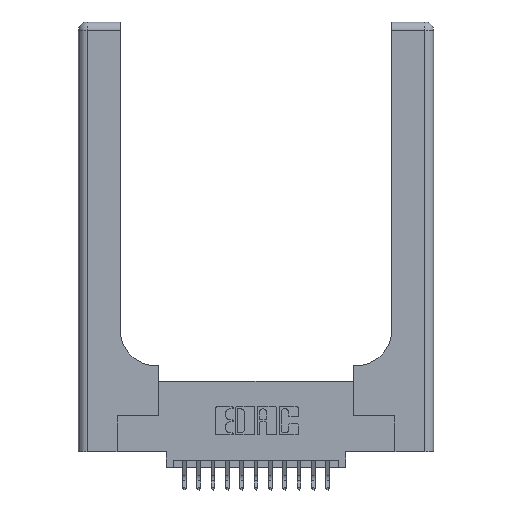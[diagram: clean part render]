
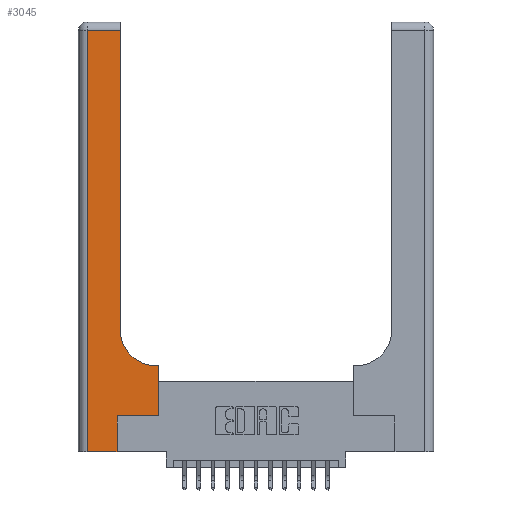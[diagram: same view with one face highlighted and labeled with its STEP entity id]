
A CAD part, top view. The second image highlights one B-rep face of the part: STEP entity #3045.
In plain terms, the highlighted planar face has unit normal (0, 0, 1).
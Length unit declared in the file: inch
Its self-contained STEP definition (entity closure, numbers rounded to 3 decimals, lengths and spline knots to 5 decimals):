
#62 = EDGE_CURVE ( 'NONE', #556, #14272, #10894, .T. ) ;
#209 = ORIENTED_EDGE ( 'NONE', *, *, #3228, .T. ) ;
#393 = ORIENTED_EDGE ( 'NONE', *, *, #5946, .T. ) ;
#556 = VERTEX_POINT ( 'NONE', #5649 ) ;
#720 = VERTEX_POINT ( 'NONE', #1015 ) ;
#737 = CARTESIAN_POINT ( 'NONE',  ( 0.269, 0.25, 0.37 ) ) ;
#1014 = LINE ( 'NONE', #6692, #4306 ) ;
#1015 = CARTESIAN_POINT ( 'NONE',  ( 0.5415, 0.6, 0.37 ) ) ;
#1060 = CARTESIAN_POINT ( 'NONE',  ( 0.06, 0., 0.37 ) ) ;
#1127 = CARTESIAN_POINT ( 'NONE',  ( 0., 3., 0.37 ) ) ;
#1320 = DIRECTION ( 'NONE',  ( -1., 0., 0. ) ) ;
#1428 = ORIENTED_EDGE ( 'NONE', *, *, #4785, .T. ) ;
#1470 = CARTESIAN_POINT ( 'NONE',  ( 0., 2.94, 0.37 ) ) ;
#2487 = LINE ( 'NONE', #14448, #9619 ) ;
#2597 = VECTOR ( 'NONE', #16921, 39.37008 ) ;
#3045 = ADVANCED_FACE ( 'NONE', ( #12782 ), #7620, .F. ) ;
#3191 = DIRECTION ( 'NONE',  ( 0., 1., 0. ) ) ;
#3228 = EDGE_CURVE ( 'NONE', #4507, #6204, #1014, .T. ) ;
#3285 = DIRECTION ( 'NONE',  ( 1., 0., 0. ) ) ;
#3406 = VECTOR ( 'NONE', #9528, 39.37008 ) ;
#3554 = ORIENTED_EDGE ( 'NONE', *, *, #9124, .T. ) ;
#3747 = LINE ( 'NONE', #6842, #15785 ) ;
#3970 = CARTESIAN_POINT ( 'NONE',  ( 0.2915, 0.85, 0.37 ) ) ;
#4130 = CARTESIAN_POINT ( 'NONE',  ( 0.269, 0., 0.37 ) ) ;
#4306 = VECTOR ( 'NONE', #12244, 39.37008 ) ;
#4507 = VERTEX_POINT ( 'NONE', #10800 ) ;
#4729 = LINE ( 'NONE', #10486, #10089 ) ;
#4785 = EDGE_CURVE ( 'NONE', #6204, #15119, #2487, .T. ) ;
#4969 = ORIENTED_EDGE ( 'NONE', *, *, #13671, .T. ) ;
#5626 = DIRECTION ( 'NONE',  ( 0., 0., -1. ) ) ;
#5649 = CARTESIAN_POINT ( 'NONE',  ( 0.269, 0.25, 0.37 ) ) ;
#5757 = CIRCLE ( 'NONE', #16967, 0.25 ) ;
#5946 = EDGE_CURVE ( 'NONE', #11064, #14195, #4729, .T. ) ;
#6022 = EDGE_LOOP ( 'NONE', ( #393, #6924, #209, #1428, #7996, #14332, #7759, #4969, #3554 ) ) ;
#6204 = VERTEX_POINT ( 'NONE', #1060 ) ;
#6692 = CARTESIAN_POINT ( 'NONE',  ( 0.06, 3., 0.37 ) ) ;
#6842 = CARTESIAN_POINT ( 'NONE',  ( 0.2915, 0.6, 0.37 ) ) ;
#6924 = ORIENTED_EDGE ( 'NONE', *, *, #10395, .T. ) ;
#7087 = VECTOR ( 'NONE', #14965, 39.37008 ) ;
#7620 = PLANE ( 'NONE',  #17017 ) ;
#7759 = ORIENTED_EDGE ( 'NONE', *, *, #17238, .T. ) ;
#7996 = ORIENTED_EDGE ( 'NONE', *, *, #16711, .T. ) ;
#9124 = EDGE_CURVE ( 'NONE', #720, #11064, #5757, .T. ) ;
#9528 = DIRECTION ( 'NONE',  ( 0., 1., 0. ) ) ;
#9619 = VECTOR ( 'NONE', #3285, 39.37008 ) ;
#10089 = VECTOR ( 'NONE', #11914, 39.37008 ) ;
#10395 = EDGE_CURVE ( 'NONE', #14195, #4507, #17939, .T. ) ;
#10486 = CARTESIAN_POINT ( 'NONE',  ( 0.2915, 3., 0.37 ) ) ;
#10800 = CARTESIAN_POINT ( 'NONE',  ( 0.06, 2.94, 0.37 ) ) ;
#10894 = LINE ( 'NONE', #737, #7087 ) ;
#11064 = VERTEX_POINT ( 'NONE', #3970 ) ;
#11742 = CARTESIAN_POINT ( 'NONE',  ( 0.5585, 0.25, 0.37 ) ) ;
#11914 = DIRECTION ( 'NONE',  ( 0., 1., 0. ) ) ;
#12244 = DIRECTION ( 'NONE',  ( 0., -1., 0. ) ) ;
#12433 = DIRECTION ( 'NONE',  ( 0., 0., -1. ) ) ;
#12497 = DIRECTION ( 'NONE',  ( 1., 0., 0. ) ) ;
#12782 = FACE_OUTER_BOUND ( 'NONE', #6022, .T. ) ;
#12825 = VERTEX_POINT ( 'NONE', #13288 ) ;
#13288 = CARTESIAN_POINT ( 'NONE',  ( 0.5585, 0.6, 0.37 ) ) ;
#13458 = LINE ( 'NONE', #17753, #3406 ) ;
#13671 = EDGE_CURVE ( 'NONE', #12825, #720, #3747, .T. ) ;
#13675 = CARTESIAN_POINT ( 'NONE',  ( 0.2915, 2.94, 0.37 ) ) ;
#14195 = VERTEX_POINT ( 'NONE', #13675 ) ;
#14272 = VERTEX_POINT ( 'NONE', #18236 ) ;
#14332 = ORIENTED_EDGE ( 'NONE', *, *, #62, .T. ) ;
#14448 = CARTESIAN_POINT ( 'NONE',  ( 0., 0., 0.37 ) ) ;
#14777 = VECTOR ( 'NONE', #3191, 39.37008 ) ;
#14965 = DIRECTION ( 'NONE',  ( 1., 0., 0. ) ) ;
#15119 = VERTEX_POINT ( 'NONE', #4130 ) ;
#15454 = DIRECTION ( 'NONE',  ( -1., 0., 0. ) ) ;
#15785 = VECTOR ( 'NONE', #1320, 39.37008 ) ;
#16711 = EDGE_CURVE ( 'NONE', #15119, #556, #13458, .T. ) ;
#16921 = DIRECTION ( 'NONE',  ( -1., 0., 0. ) ) ;
#16967 = AXIS2_PLACEMENT_3D ( 'NONE', #18001, #12433, #12497 ) ;
#17017 = AXIS2_PLACEMENT_3D ( 'NONE', #1127, #5626, #15454 ) ;
#17238 = EDGE_CURVE ( 'NONE', #14272, #12825, #17419, .T. ) ;
#17419 = LINE ( 'NONE', #11742, #14777 ) ;
#17753 = CARTESIAN_POINT ( 'NONE',  ( 0.269, 0., 0.37 ) ) ;
#17939 = LINE ( 'NONE', #1470, #2597 ) ;
#18001 = CARTESIAN_POINT ( 'NONE',  ( 0.5415, 0.85, 0.37 ) ) ;
#18236 = CARTESIAN_POINT ( 'NONE',  ( 0.5585, 0.25, 0.37 ) ) ;
